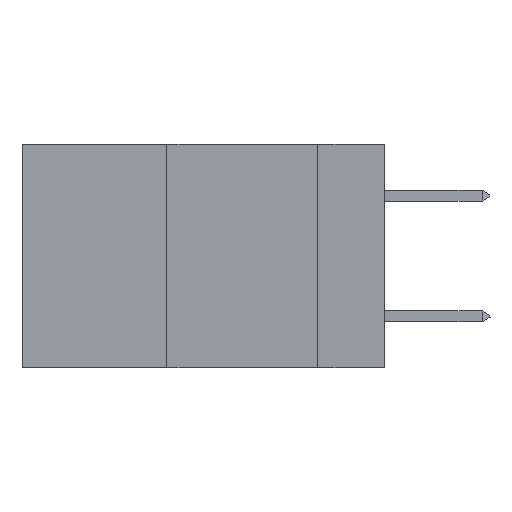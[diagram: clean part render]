
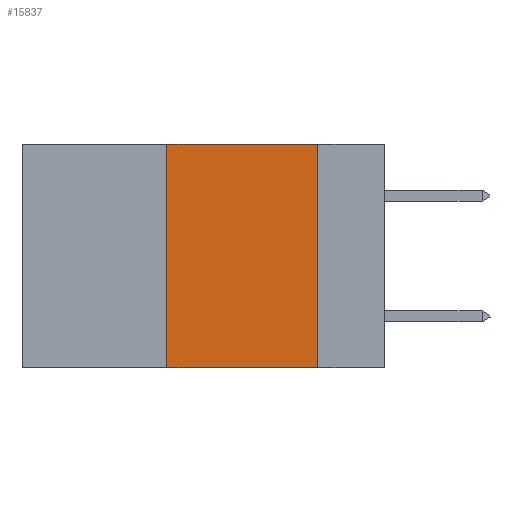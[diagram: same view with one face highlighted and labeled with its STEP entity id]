
A CAD part, left-side view. The second image highlights one B-rep face of the part: STEP entity #15837.
In plain terms, the highlighted planar face has unit normal (-1, 0, 0).
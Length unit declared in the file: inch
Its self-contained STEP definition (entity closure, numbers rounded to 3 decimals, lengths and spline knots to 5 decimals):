
#19 = VECTOR ( 'NONE', #11336, 39.37008 ) ;
#68 = FACE_OUTER_BOUND ( 'NONE', #15839, .T. ) ;
#1644 = EDGE_CURVE ( 'NONE', #8054, #3723, #14480, .T. ) ;
#2518 = ORIENTED_EDGE ( 'NONE', *, *, #20448, .T. ) ;
#3723 = VERTEX_POINT ( 'NONE', #19795 ) ;
#3942 = VECTOR ( 'NONE', #21219, 39.37008 ) ;
#5298 = DIRECTION ( 'NONE',  ( 0., -1., 0. ) ) ;
#6467 = DIRECTION ( 'NONE',  ( 0., 0., -1. ) ) ;
#7568 = CARTESIAN_POINT ( 'NONE',  ( 0., 0.36, 0. ) ) ;
#8054 = VERTEX_POINT ( 'NONE', #21572 ) ;
#9827 = ORIENTED_EDGE ( 'NONE', *, *, #20236, .F. ) ;
#9930 = PLANE ( 'NONE',  #10920 ) ;
#10013 = DIRECTION ( 'NONE',  ( 1., 0., 0. ) ) ;
#10096 = CARTESIAN_POINT ( 'NONE',  ( 0., 0.11, 0. ) ) ;
#10362 = LINE ( 'NONE', #22408, #16588 ) ;
#10920 = AXIS2_PLACEMENT_3D ( 'NONE', #13406, #10013, #6467 ) ;
#11336 = DIRECTION ( 'NONE',  ( 0., 0., 1. ) ) ;
#12040 = VECTOR ( 'NONE', #5298, 39.37008 ) ;
#13406 = CARTESIAN_POINT ( 'NONE',  ( 0., 0.6, 0. ) ) ;
#14104 = VERTEX_POINT ( 'NONE', #20043 ) ;
#14480 = LINE ( 'NONE', #7568, #19 ) ;
#14975 = DIRECTION ( 'NONE',  ( 0., -1., 0. ) ) ;
#15837 = ADVANCED_FACE ( 'NONE', ( #68 ), #9930, .F. ) ;
#15839 = EDGE_LOOP ( 'NONE', ( #16415, #9827, #23053, #2518 ) ) ;
#16415 = ORIENTED_EDGE ( 'NONE', *, *, #17987, .F. ) ;
#16588 = VECTOR ( 'NONE', #14975, 39.37008 ) ;
#17987 = EDGE_CURVE ( 'NONE', #14104, #19996, #21844, .T. ) ;
#19462 = LINE ( 'NONE', #21295, #12040 ) ;
#19795 = CARTESIAN_POINT ( 'NONE',  ( 0., 0.36, 0. ) ) ;
#19996 = VERTEX_POINT ( 'NONE', #22265 ) ;
#20043 = CARTESIAN_POINT ( 'NONE',  ( 0., 0.11, 0. ) ) ;
#20236 = EDGE_CURVE ( 'NONE', #3723, #14104, #19462, .T. ) ;
#20448 = EDGE_CURVE ( 'NONE', #8054, #19996, #10362, .T. ) ;
#21219 = DIRECTION ( 'NONE',  ( 0., 0., -1. ) ) ;
#21295 = CARTESIAN_POINT ( 'NONE',  ( 0., 0.6, 0. ) ) ;
#21572 = CARTESIAN_POINT ( 'NONE',  ( 0., 0.36, -0.37 ) ) ;
#21844 = LINE ( 'NONE', #10096, #3942 ) ;
#22265 = CARTESIAN_POINT ( 'NONE',  ( 0., 0.11, -0.37 ) ) ;
#22408 = CARTESIAN_POINT ( 'NONE',  ( 0., 0.6, -0.37 ) ) ;
#23053 = ORIENTED_EDGE ( 'NONE', *, *, #1644, .F. ) ;
